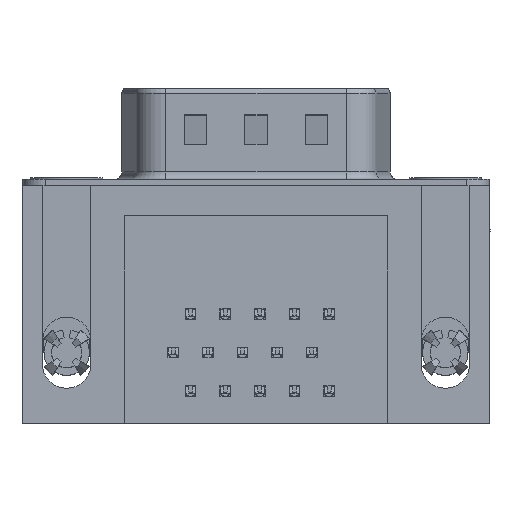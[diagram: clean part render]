
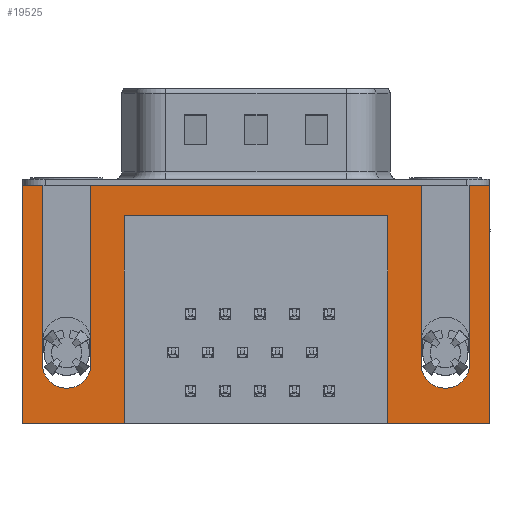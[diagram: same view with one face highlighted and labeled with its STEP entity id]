
A CAD part, front view. The second image highlights one B-rep face of the part: STEP entity #19525.
In plain terms, the highlighted planar face has unit normal (0, -1, 0).
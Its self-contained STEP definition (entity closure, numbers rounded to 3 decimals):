
#12 = VERTEX_POINT ( 'NONE', #4478 ) ;
#727 = ORIENTED_EDGE ( 'NONE', *, *, #1726, .F. ) ;
#927 = VERTEX_POINT ( 'NONE', #20187 ) ;
#985 = CIRCLE ( 'NONE', #12458, 1.6 ) ;
#998 = ORIENTED_EDGE ( 'NONE', *, *, #18933, .F. ) ;
#1034 = CARTESIAN_POINT ( 'NONE',  ( 26.59, -6.275, 0. ) ) ;
#1064 = VERTEX_POINT ( 'NONE', #12763 ) ;
#1280 = LINE ( 'NONE', #2057, #14571 ) ;
#1343 = CARTESIAN_POINT ( 'NONE',  ( -2.91, -6.275, -2.5 ) ) ;
#1383 = VERTEX_POINT ( 'NONE', #18353 ) ;
#1446 = ORIENTED_EDGE ( 'NONE', *, *, #7692, .F. ) ;
#1506 = DIRECTION ( 'NONE',  ( 0., 0., 1. ) ) ;
#1595 = VECTOR ( 'NONE', #4764, 1000. ) ;
#1629 = VERTEX_POINT ( 'NONE', #14564 ) ;
#1726 = EDGE_CURVE ( 'NONE', #6456, #15048, #985, .T. ) ;
#2057 = CARTESIAN_POINT ( 'NONE',  ( -2.91, -6.275, 0. ) ) ;
#2270 = CARTESIAN_POINT ( 'NONE',  ( 24.99, -6.275, -11.78 ) ) ;
#2293 = EDGE_CURVE ( 'NONE', #12, #15067, #3745, .T. ) ;
#2344 = CARTESIAN_POINT ( 'NONE',  ( 3.79, -6.275, -2. ) ) ;
#2398 = VECTOR ( 'NONE', #15925, 1000. ) ;
#2574 = ORIENTED_EDGE ( 'NONE', *, *, #11012, .F. ) ;
#2608 = ORIENTED_EDGE ( 'NONE', *, *, #3299, .F. ) ;
#2960 = CARTESIAN_POINT ( 'NONE',  ( 24.99, -6.275, -11.78 ) ) ;
#3006 = CARTESIAN_POINT ( 'NONE',  ( 0., -6.275, -11.78 ) ) ;
#3117 = DIRECTION ( 'NONE',  ( 0., 0., -1. ) ) ;
#3299 = EDGE_CURVE ( 'NONE', #15048, #4881, #18071, .T. ) ;
#3329 = DIRECTION ( 'NONE',  ( -1., 0., 0. ) ) ;
#3399 = VERTEX_POINT ( 'NONE', #14947 ) ;
#3528 = LINE ( 'NONE', #6031, #11779 ) ;
#3531 = CIRCLE ( 'NONE', #4322, 1.6 ) ;
#3578 = DIRECTION ( 'NONE',  ( 0., 0., 1. ) ) ;
#3742 = LINE ( 'NONE', #9013, #16372 ) ;
#3745 = LINE ( 'NONE', #17691, #12482 ) ;
#3801 = CARTESIAN_POINT ( 'NONE',  ( 21.2, -6.275, -2. ) ) ;
#3843 = VERTEX_POINT ( 'NONE', #15891 ) ;
#4028 = DIRECTION ( 'NONE',  ( 0., 0., 1. ) ) ;
#4136 = LINE ( 'NONE', #9835, #21210 ) ;
#4322 = AXIS2_PLACEMENT_3D ( 'NONE', #2270, #13844, #4028 ) ;
#4420 = CARTESIAN_POINT ( 'NONE',  ( 23.39, -6.275, 0. ) ) ;
#4478 = CARTESIAN_POINT ( 'NONE',  ( 27.9, -6.275, -15.7 ) ) ;
#4698 = DIRECTION ( 'NONE',  ( 0., 0., 1. ) ) ;
#4716 = VERTEX_POINT ( 'NONE', #14360 ) ;
#4764 = DIRECTION ( 'NONE',  ( -1., 0., 0. ) ) ;
#4881 = VERTEX_POINT ( 'NONE', #13601 ) ;
#5201 = ORIENTED_EDGE ( 'NONE', *, *, #19006, .F. ) ;
#5470 = EDGE_CURVE ( 'NONE', #15067, #1064, #13116, .T. ) ;
#6031 = CARTESIAN_POINT ( 'NONE',  ( -2.91, -6.275, 0. ) ) ;
#6249 = DIRECTION ( 'NONE',  ( 1., 0., 0. ) ) ;
#6356 = VECTOR ( 'NONE', #1506, 1000. ) ;
#6456 = VERTEX_POINT ( 'NONE', #19749 ) ;
#6806 = VECTOR ( 'NONE', #6249, 1000. ) ;
#6894 = LINE ( 'NONE', #21478, #6356 ) ;
#6926 = LINE ( 'NONE', #4420, #2398 ) ;
#6945 = VECTOR ( 'NONE', #12260, 1000. ) ;
#7117 = ORIENTED_EDGE ( 'NONE', *, *, #15601, .F. ) ;
#7290 = CARTESIAN_POINT ( 'NONE',  ( 3.79, -6.275, -2. ) ) ;
#7383 = LINE ( 'NONE', #1034, #7916 ) ;
#7409 = DIRECTION ( 'NONE',  ( 0., 0., -1. ) ) ;
#7692 = EDGE_CURVE ( 'NONE', #1383, #6456, #18264, .T. ) ;
#7718 = DIRECTION ( 'NONE',  ( 1., 0., 0. ) ) ;
#7888 = VERTEX_POINT ( 'NONE', #19279 ) ;
#7916 = VECTOR ( 'NONE', #21016, 1000. ) ;
#7989 = ORIENTED_EDGE ( 'NONE', *, *, #10978, .F. ) ;
#8150 = CARTESIAN_POINT ( 'NONE',  ( -2.91, -6.275, -2.5 ) ) ;
#8479 = VERTEX_POINT ( 'NONE', #20720 ) ;
#8783 = EDGE_CURVE ( 'NONE', #1064, #9519, #4136, .T. ) ;
#8962 = DIRECTION ( 'NONE',  ( 0., -1., 0. ) ) ;
#9013 = CARTESIAN_POINT ( 'NONE',  ( -1.6, -6.275, 0. ) ) ;
#9462 = ORIENTED_EDGE ( 'NONE', *, *, #21133, .F. ) ;
#9519 = VERTEX_POINT ( 'NONE', #7290 ) ;
#9530 = CARTESIAN_POINT ( 'NONE',  ( 1.6, -6.275, -11.78 ) ) ;
#9789 = FACE_OUTER_BOUND ( 'NONE', #20109, .T. ) ;
#9835 = CARTESIAN_POINT ( 'NONE',  ( 3.79, -6.275, -2. ) ) ;
#10090 = LINE ( 'NONE', #8150, #13917 ) ;
#10978 = EDGE_CURVE ( 'NONE', #8479, #3843, #3531, .T. ) ;
#11012 = EDGE_CURVE ( 'NONE', #9519, #13482, #15651, .T. ) ;
#11120 = LINE ( 'NONE', #12741, #6806 ) ;
#11138 = AXIS2_PLACEMENT_3D ( 'NONE', #18744, #8962, #20514 ) ;
#11327 = EDGE_CURVE ( 'NONE', #13482, #927, #18652, .T. ) ;
#11779 = VECTOR ( 'NONE', #7718, 1000. ) ;
#11997 = DIRECTION ( 'NONE',  ( 1., 0., 0. ) ) ;
#12260 = DIRECTION ( 'NONE',  ( 0., 0., -1. ) ) ;
#12458 = AXIS2_PLACEMENT_3D ( 'NONE', #3006, #13135, #12892 ) ;
#12482 = VECTOR ( 'NONE', #3329, 1000. ) ;
#12741 = CARTESIAN_POINT ( 'NONE',  ( -2.91, -6.275, 0. ) ) ;
#12763 = CARTESIAN_POINT ( 'NONE',  ( 21.2, -6.275, -2. ) ) ;
#12892 = DIRECTION ( 'NONE',  ( 0., 0., -1. ) ) ;
#12947 = ORIENTED_EDGE ( 'NONE', *, *, #21063, .F. ) ;
#12961 = DIRECTION ( 'NONE',  ( 0., 0., 1. ) ) ;
#13003 = DIRECTION ( 'NONE',  ( 0., -1., 0. ) ) ;
#13116 = LINE ( 'NONE', #3801, #16949 ) ;
#13135 = DIRECTION ( 'NONE',  ( 0., -1., 0. ) ) ;
#13277 = EDGE_CURVE ( 'NONE', #3843, #7888, #7383, .T. ) ;
#13346 = EDGE_CURVE ( 'NONE', #18733, #8479, #18858, .T. ) ;
#13482 = VERTEX_POINT ( 'NONE', #19702 ) ;
#13601 = CARTESIAN_POINT ( 'NONE',  ( 1.6, -6.275, 0. ) ) ;
#13635 = DIRECTION ( 'NONE',  ( 0., 0., 1. ) ) ;
#13844 = DIRECTION ( 'NONE',  ( 0., -1., 0. ) ) ;
#13917 = VECTOR ( 'NONE', #12961, 1000. ) ;
#14177 = CARTESIAN_POINT ( 'NONE',  ( 23.39, -6.275, 0. ) ) ;
#14247 = AXIS2_PLACEMENT_3D ( 'NONE', #2960, #14518, #4698 ) ;
#14360 = CARTESIAN_POINT ( 'NONE',  ( 27.9, -6.275, 0. ) ) ;
#14518 = DIRECTION ( 'NONE',  ( 0., -1., 0. ) ) ;
#14564 = CARTESIAN_POINT ( 'NONE',  ( -2.91, -6.275, 0. ) ) ;
#14571 = VECTOR ( 'NONE', #11997, 1000. ) ;
#14598 = PLANE ( 'NONE',  #17894 ) ;
#14744 = ORIENTED_EDGE ( 'NONE', *, *, #21421, .T. ) ;
#14795 = ORIENTED_EDGE ( 'NONE', *, *, #16107, .F. ) ;
#14947 = CARTESIAN_POINT ( 'NONE',  ( -1.6, -6.275, 0. ) ) ;
#15048 = VERTEX_POINT ( 'NONE', #9530 ) ;
#15067 = VERTEX_POINT ( 'NONE', #19384 ) ;
#15358 = ORIENTED_EDGE ( 'NONE', *, *, #2293, .F. ) ;
#15434 = CARTESIAN_POINT ( 'NONE',  ( 23.39, -6.275, -11.78 ) ) ;
#15601 = EDGE_CURVE ( 'NONE', #1629, #3399, #3528, .T. ) ;
#15651 = LINE ( 'NONE', #2344, #6945 ) ;
#15891 = CARTESIAN_POINT ( 'NONE',  ( 26.59, -6.275, -11.78 ) ) ;
#15925 = DIRECTION ( 'NONE',  ( 0., 0., -1. ) ) ;
#16107 = EDGE_CURVE ( 'NONE', #17093, #18733, #6926, .T. ) ;
#16372 = VECTOR ( 'NONE', #7409, 1000. ) ;
#16396 = DIRECTION ( 'NONE',  ( -1., 0., 0. ) ) ;
#16911 = ORIENTED_EDGE ( 'NONE', *, *, #13346, .F. ) ;
#16949 = VECTOR ( 'NONE', #13635, 1000. ) ;
#17093 = VERTEX_POINT ( 'NONE', #14177 ) ;
#17557 = VECTOR ( 'NONE', #3578, 1000. ) ;
#17691 = CARTESIAN_POINT ( 'NONE',  ( 27.9, -6.275, -15.7 ) ) ;
#17894 = AXIS2_PLACEMENT_3D ( 'NONE', #1343, #13003, #3117 ) ;
#18071 = LINE ( 'NONE', #19502, #17557 ) ;
#18264 = CIRCLE ( 'NONE', #11138, 1.6 ) ;
#18353 = CARTESIAN_POINT ( 'NONE',  ( -1.6, -6.275, -11.78 ) ) ;
#18652 = LINE ( 'NONE', #21318, #1595 ) ;
#18733 = VERTEX_POINT ( 'NONE', #15434 ) ;
#18744 = CARTESIAN_POINT ( 'NONE',  ( 0., -6.275, -11.78 ) ) ;
#18858 = CIRCLE ( 'NONE', #14247, 1.6 ) ;
#18933 = EDGE_CURVE ( 'NONE', #4881, #17093, #11120, .T. ) ;
#19006 = EDGE_CURVE ( 'NONE', #927, #1629, #10090, .T. ) ;
#19279 = CARTESIAN_POINT ( 'NONE',  ( 26.59, -6.275, 0. ) ) ;
#19348 = ORIENTED_EDGE ( 'NONE', *, *, #5470, .F. ) ;
#19384 = CARTESIAN_POINT ( 'NONE',  ( 21.2, -6.275, -15.7 ) ) ;
#19502 = CARTESIAN_POINT ( 'NONE',  ( 1.6, -6.275, 0. ) ) ;
#19525 = ADVANCED_FACE ( 'NONE', ( #9789 ), #14598, .T. ) ;
#19702 = CARTESIAN_POINT ( 'NONE',  ( 3.79, -6.275, -15.7 ) ) ;
#19749 = CARTESIAN_POINT ( 'NONE',  ( 0., -6.275, -13.38 ) ) ;
#19837 = ORIENTED_EDGE ( 'NONE', *, *, #13277, .F. ) ;
#20109 = EDGE_LOOP ( 'NONE', ( #19837, #7989, #16911, #14795, #998, #2608, #727, #1446, #9462, #7117, #5201, #20405, #2574, #20551, #19348, #15358, #14744, #12947 ) ) ;
#20187 = CARTESIAN_POINT ( 'NONE',  ( -2.91, -6.275, -15.7 ) ) ;
#20405 = ORIENTED_EDGE ( 'NONE', *, *, #11327, .F. ) ;
#20514 = DIRECTION ( 'NONE',  ( 0., 0., -1. ) ) ;
#20551 = ORIENTED_EDGE ( 'NONE', *, *, #8783, .F. ) ;
#20720 = CARTESIAN_POINT ( 'NONE',  ( 24.99, -6.275, -13.38 ) ) ;
#21016 = DIRECTION ( 'NONE',  ( 0., 0., 1. ) ) ;
#21063 = EDGE_CURVE ( 'NONE', #7888, #4716, #1280, .T. ) ;
#21133 = EDGE_CURVE ( 'NONE', #3399, #1383, #3742, .T. ) ;
#21210 = VECTOR ( 'NONE', #16396, 1000. ) ;
#21318 = CARTESIAN_POINT ( 'NONE',  ( 27.9, -6.275, -15.7 ) ) ;
#21421 = EDGE_CURVE ( 'NONE', #12, #4716, #6894, .T. ) ;
#21478 = CARTESIAN_POINT ( 'NONE',  ( 27.9, -6.275, -2.5 ) ) ;
